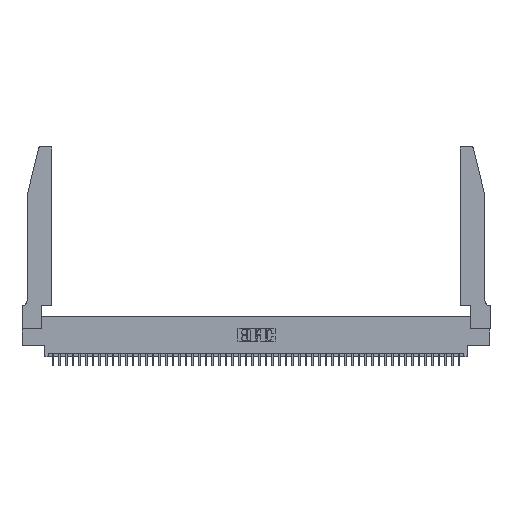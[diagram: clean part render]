
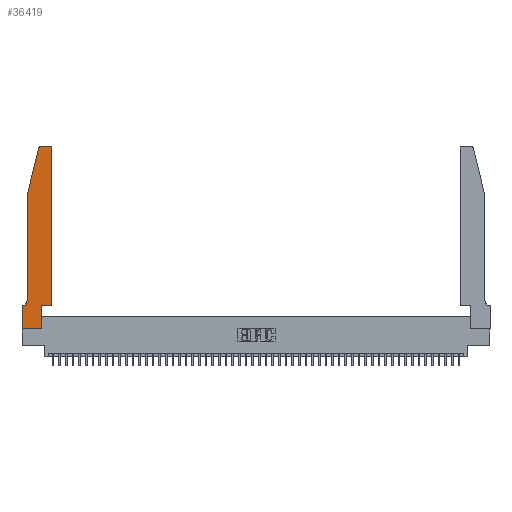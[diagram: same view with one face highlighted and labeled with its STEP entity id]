
A CAD part, top view. The second image highlights one B-rep face of the part: STEP entity #36419.
In plain terms, the highlighted planar face has unit normal (0, 0, 1).
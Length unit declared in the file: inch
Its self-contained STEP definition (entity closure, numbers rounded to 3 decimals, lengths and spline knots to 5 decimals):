
#1155 = VERTEX_POINT ( 'NONE', #18152 ) ;
#1391 = CARTESIAN_POINT ( 'NONE',  ( 0.4205, 2.72, 0.37 ) ) ;
#2303 = CARTESIAN_POINT ( 'NONE',  ( 0.4505, 0.35, 0.37 ) ) ;
#2352 = CARTESIAN_POINT ( 'NONE',  ( 0.4505, 0.35, 0.37 ) ) ;
#2548 = VECTOR ( 'NONE', #23670, 39.37008 ) ;
#2700 = VECTOR ( 'NONE', #23134, 39.37008 ) ;
#3422 = EDGE_CURVE ( 'NONE', #7166, #26334, #14384, .T. ) ;
#3714 = EDGE_CURVE ( 'NONE', #10741, #38900, #17049, .T. ) ;
#4539 = CARTESIAN_POINT ( 'NONE',  ( 0.2865, 0.35, 0.37 ) ) ;
#5279 = VERTEX_POINT ( 'NONE', #30725 ) ;
#5364 = AXIS2_PLACEMENT_3D ( 'NONE', #41613, #29967, #6346 ) ;
#5409 = DIRECTION ( 'NONE',  ( 1., 0., 0. ) ) ;
#5558 = ORIENTED_EDGE ( 'NONE', *, *, #3714, .T. ) ;
#5598 = VERTEX_POINT ( 'NONE', #36512 ) ;
#5993 = VECTOR ( 'NONE', #12585, 39.37008 ) ;
#6004 = CARTESIAN_POINT ( 'NONE',  ( 0.284, 2.72, 0.37 ) ) ;
#6346 = DIRECTION ( 'NONE',  ( 1., 0., 0. ) ) ;
#7166 = VERTEX_POINT ( 'NONE', #14607 ) ;
#7265 = VECTOR ( 'NONE', #46430, 39.37008 ) ;
#7273 = EDGE_CURVE ( 'NONE', #5598, #1155, #18978, .T. ) ;
#7402 = DIRECTION ( 'NONE',  ( 1., 0., 0. ) ) ;
#7426 = CARTESIAN_POINT ( 'NONE',  ( 0.0055, 0.42, 0.37 ) ) ;
#8109 = LINE ( 'NONE', #34949, #38221 ) ;
#9084 = AXIS2_PLACEMENT_3D ( 'NONE', #7426, #34961, #11435 ) ;
#9737 = ORIENTED_EDGE ( 'NONE', *, *, #29183, .T. ) ;
#10037 = DIRECTION ( 'NONE',  ( 1., 0., 0. ) ) ;
#10208 = CARTESIAN_POINT ( 'NONE',  ( 0.25487, 2.72718, 0.37 ) ) ;
#10337 = DIRECTION ( 'NONE',  ( 0., 1., 0. ) ) ;
#10741 = VERTEX_POINT ( 'NONE', #35780 ) ;
#11435 = DIRECTION ( 'NONE',  ( -1., 0., 0. ) ) ;
#12000 = CARTESIAN_POINT ( 'NONE',  ( 0.0755, 2., 0.37 ) ) ;
#12044 = EDGE_CURVE ( 'NONE', #33953, #24997, #37407, .T. ) ;
#12278 = ORIENTED_EDGE ( 'NONE', *, *, #7273, .T. ) ;
#12585 = DIRECTION ( 'NONE',  ( 0., 1., 0. ) ) ;
#13099 = EDGE_CURVE ( 'NONE', #26334, #5598, #41582, .T. ) ;
#14173 = ORIENTED_EDGE ( 'NONE', *, *, #24022, .T. ) ;
#14384 = LINE ( 'NONE', #12000, #2548 ) ;
#14607 = CARTESIAN_POINT ( 'NONE',  ( 0.0755, 2., 0.37 ) ) ;
#14834 = DIRECTION ( 'NONE',  ( -1., 0., 0. ) ) ;
#15152 = ORIENTED_EDGE ( 'NONE', *, *, #30531, .T. ) ;
#16848 = EDGE_CURVE ( 'NONE', #24997, #17881, #8109, .T. ) ;
#17049 = CIRCLE ( 'NONE', #37124, 0.03 ) ;
#17718 = VECTOR ( 'NONE', #46335, 39.37008 ) ;
#17881 = VERTEX_POINT ( 'NONE', #2352 ) ;
#18152 = CARTESIAN_POINT ( 'NONE',  ( 0., 0.35, 0.37 ) ) ;
#18184 = VECTOR ( 'NONE', #20925, 39.37008 ) ;
#18622 = CARTESIAN_POINT ( 'NONE',  ( 0.2865, 0.35, 0.37 ) ) ;
#18924 = VERTEX_POINT ( 'NONE', #36225 ) ;
#18978 = LINE ( 'NONE', #42557, #7265 ) ;
#20925 = DIRECTION ( 'NONE',  ( 0., -1., 0. ) ) ;
#22272 = CIRCLE ( 'NONE', #32506, 0.03 ) ;
#23134 = DIRECTION ( 'NONE',  ( 1., 0., 0. ) ) ;
#23670 = DIRECTION ( 'NONE',  ( 0., -1., 0. ) ) ;
#23933 = EDGE_LOOP ( 'NONE', ( #50862, #5558, #9737, #34892, #31452, #12278, #14173, #15152, #25365, #47947, #43841, #49817 ) ) ;
#24022 = EDGE_CURVE ( 'NONE', #1155, #5279, #39071, .T. ) ;
#24958 = LINE ( 'NONE', #50301, #2700 ) ;
#24997 = VERTEX_POINT ( 'NONE', #18622 ) ;
#25365 = ORIENTED_EDGE ( 'NONE', *, *, #12044, .T. ) ;
#25592 = EDGE_CURVE ( 'NONE', #18924, #10741, #39526, .T. ) ;
#25617 = CARTESIAN_POINT ( 'NONE',  ( 0.4505, 2.72, 0.37 ) ) ;
#26021 = EDGE_CURVE ( 'NONE', #29583, #18924, #22272, .T. ) ;
#26334 = VERTEX_POINT ( 'NONE', #29944 ) ;
#26470 = FACE_OUTER_BOUND ( 'NONE', #23933, .T. ) ;
#29045 = DIRECTION ( 'NONE',  ( 0., 0., 1. ) ) ;
#29183 = EDGE_CURVE ( 'NONE', #38900, #7166, #48930, .T. ) ;
#29583 = VERTEX_POINT ( 'NONE', #25617 ) ;
#29944 = CARTESIAN_POINT ( 'NONE',  ( 0.0755, 0.42, 0.37 ) ) ;
#29967 = DIRECTION ( 'NONE',  ( 0., 0., 1. ) ) ;
#30531 = EDGE_CURVE ( 'NONE', #5279, #33953, #24958, .T. ) ;
#30725 = CARTESIAN_POINT ( 'NONE',  ( 0., 0., 0.37 ) ) ;
#31452 = ORIENTED_EDGE ( 'NONE', *, *, #13099, .T. ) ;
#32506 = AXIS2_PLACEMENT_3D ( 'NONE', #1391, #29045, #5409 ) ;
#33577 = DIRECTION ( 'NONE',  ( 0., 0., 1. ) ) ;
#33953 = VERTEX_POINT ( 'NONE', #45224 ) ;
#34892 = ORIENTED_EDGE ( 'NONE', *, *, #3422, .T. ) ;
#34949 = CARTESIAN_POINT ( 'NONE',  ( 0.4505, 0.35, 0.37 ) ) ;
#34961 = DIRECTION ( 'NONE',  ( 0., 0., -1. ) ) ;
#35780 = CARTESIAN_POINT ( 'NONE',  ( 0.284, 2.75, 0.37 ) ) ;
#36225 = CARTESIAN_POINT ( 'NONE',  ( 0.4205, 2.75, 0.37 ) ) ;
#36419 = ADVANCED_FACE ( 'NONE', ( #26470 ), #45522, .T. ) ;
#36512 = CARTESIAN_POINT ( 'NONE',  ( 0.0055, 0.35, 0.37 ) ) ;
#37124 = AXIS2_PLACEMENT_3D ( 'NONE', #6004, #33577, #10037 ) ;
#37407 = LINE ( 'NONE', #4539, #5993 ) ;
#38221 = VECTOR ( 'NONE', #7402, 39.37008 ) ;
#38833 = VECTOR ( 'NONE', #10337, 39.37008 ) ;
#38900 = VERTEX_POINT ( 'NONE', #10208 ) ;
#39071 = LINE ( 'NONE', #44425, #18184 ) ;
#39526 = LINE ( 'NONE', #42260, #48635 ) ;
#41039 = EDGE_CURVE ( 'NONE', #17881, #29583, #49171, .T. ) ;
#41582 = CIRCLE ( 'NONE', #9084, 0.07 ) ;
#41613 = CARTESIAN_POINT ( 'NONE',  ( 0., 0.35, 0.37 ) ) ;
#42260 = CARTESIAN_POINT ( 'NONE',  ( 0.2605, 2.75, 0.37 ) ) ;
#42459 = CARTESIAN_POINT ( 'NONE',  ( 0.0755, 2., 0.37 ) ) ;
#42557 = CARTESIAN_POINT ( 'NONE',  ( 0.0755, 0.35, 0.37 ) ) ;
#43841 = ORIENTED_EDGE ( 'NONE', *, *, #41039, .T. ) ;
#44425 = CARTESIAN_POINT ( 'NONE',  ( 0., 0., 0.37 ) ) ;
#45224 = CARTESIAN_POINT ( 'NONE',  ( 0.2865, 0., 0.37 ) ) ;
#45522 = PLANE ( 'NONE',  #5364 ) ;
#46335 = DIRECTION ( 'NONE',  ( -0.239, -0.971, 0. ) ) ;
#46430 = DIRECTION ( 'NONE',  ( -1., 0., 0. ) ) ;
#47947 = ORIENTED_EDGE ( 'NONE', *, *, #16848, .T. ) ;
#48635 = VECTOR ( 'NONE', #14834, 39.37008 ) ;
#48930 = LINE ( 'NONE', #42459, #17718 ) ;
#49171 = LINE ( 'NONE', #2303, #38833 ) ;
#49817 = ORIENTED_EDGE ( 'NONE', *, *, #26021, .T. ) ;
#50301 = CARTESIAN_POINT ( 'NONE',  ( 0., 0., 0.37 ) ) ;
#50862 = ORIENTED_EDGE ( 'NONE', *, *, #25592, .T. ) ;
